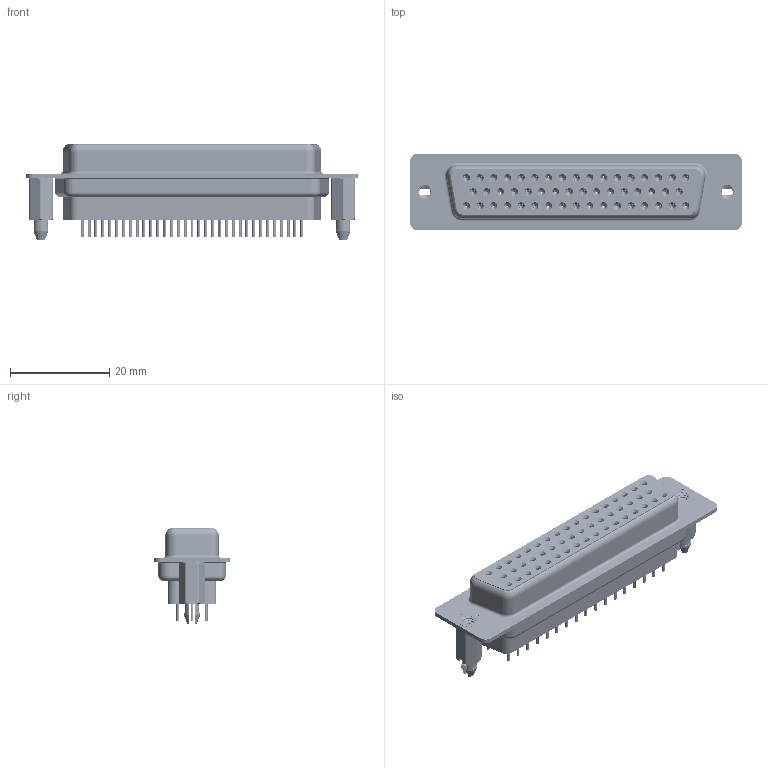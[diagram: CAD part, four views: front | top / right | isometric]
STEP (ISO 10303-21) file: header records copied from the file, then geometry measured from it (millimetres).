
FILE_DESCRIPTION (( 'STEP AP203' ), '1' );
FILE_NAME ('628-050-228-066.STEP', '2020-07-21T13:51:17', ( '' ), ( '' ), 'SwSTEP 2.0', 'SolidWorks 2020', '' );
FILE_SCHEMA (( 'CONFIG_CONTROL_DESIGN' ));
Length unit declared in the file: millimetre
Products named in the file (8): 628 Contact Row 1_28L; 628 Shell Rear_50 Contacts; 628 Shell Front_50 Contacts; 628-050-228-066; 628 Contact Row 3_28L; 628 4-40 Threaded Boardlock_FF; 628 Housing_50 FF; 628 Contact Row 2_28L
Assembly tree (55 placements, depth 2):
  628-050-228-066
    628 Housing_50 FF
    628 Shell Front_50 Contacts
    628 Shell Rear_50 Contacts
    628 Contact Row 1_28L  x17
    628 Contact Row 2_28L  x16
    628 Contact Row 3_28L  x17
    628 4-40 Threaded Boardlock_FF  x2
Bounding box: 67 x 15.4 x 19.4 mm (x, y, z)
Volume: 8030.1 mm3; surface area: 17896.3 mm2
Topology: 56 solids, 56 shells, 6896 faces, 17688 edges, 11013 vertices
Faces by surface type: cylinder 1958, plane 1655, torus 1363, bspline 1054, cone 866
Entity records: 62934 total; most frequent: CARTESIAN_POINT 26742, DIRECTION 7447, ORIENTED_EDGE 6884, EDGE_CURVE 3442, AXIS2_PLACEMENT_3D 3120, VERTEX_POINT 2195, EDGE_LOOP 1793, CIRCLE 1728
